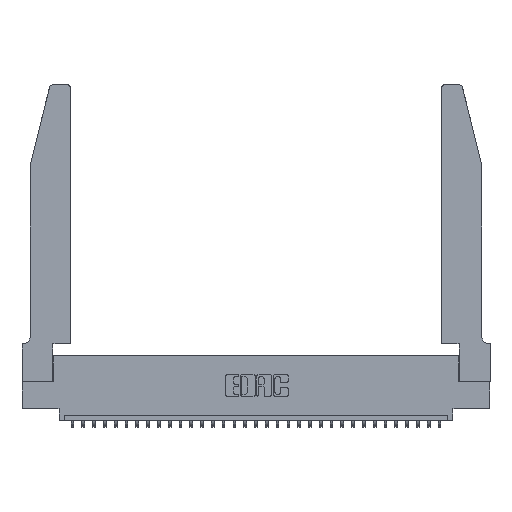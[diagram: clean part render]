
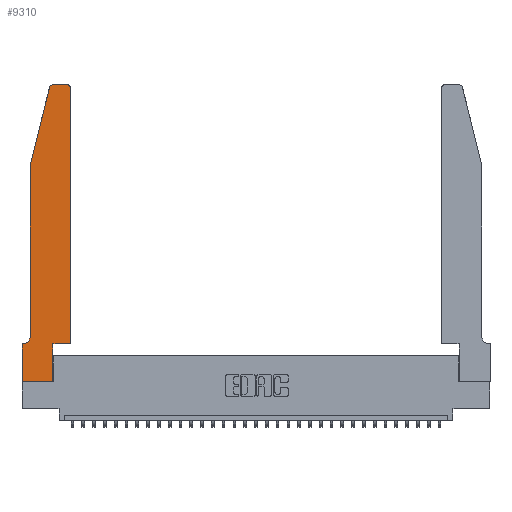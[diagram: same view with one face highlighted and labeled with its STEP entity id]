
A CAD part, top view. The second image highlights one B-rep face of the part: STEP entity #9310.
In plain terms, the highlighted planar face has unit normal (0, 0, 1).
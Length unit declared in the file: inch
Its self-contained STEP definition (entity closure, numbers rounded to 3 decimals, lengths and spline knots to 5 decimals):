
#14 = VECTOR ( 'NONE', #10910, 39.37008 ) ;
#64 = ORIENTED_EDGE ( 'NONE', *, *, #22052, .T. ) ;
#256 = VECTOR ( 'NONE', #29884, 39.37008 ) ;
#927 = DIRECTION ( 'NONE',  ( 0., 0., 1. ) ) ;
#1383 = CARTESIAN_POINT ( 'NONE',  ( 0.2865, 0.35, 0.37 ) ) ;
#1399 = VERTEX_POINT ( 'NONE', #5972 ) ;
#1616 = LINE ( 'NONE', #5135, #14 ) ;
#1634 = DIRECTION ( 'NONE',  ( -1., 0., 0. ) ) ;
#2352 = CARTESIAN_POINT ( 'NONE',  ( 0.4505, 0.35, 0.37 ) ) ;
#2363 = CIRCLE ( 'NONE', #27109, 0.03 ) ;
#3138 = CARTESIAN_POINT ( 'NONE',  ( 0.284, 2.72, 0.37 ) ) ;
#3613 = LINE ( 'NONE', #29501, #25014 ) ;
#3789 = EDGE_CURVE ( 'NONE', #22266, #21810, #1616, .T. ) ;
#3827 = DIRECTION ( 'NONE',  ( 1., 0., 0. ) ) ;
#4309 = DIRECTION ( 'NONE',  ( -0.239, -0.971, 0. ) ) ;
#4801 = EDGE_CURVE ( 'NONE', #29992, #10703, #20539, .T. ) ;
#4888 = ORIENTED_EDGE ( 'NONE', *, *, #19035, .T. ) ;
#5135 = CARTESIAN_POINT ( 'NONE',  ( 0., 0., 0.37 ) ) ;
#5917 = EDGE_CURVE ( 'NONE', #11358, #22266, #29902, .T. ) ;
#5972 = CARTESIAN_POINT ( 'NONE',  ( 0.4205, 2.75, 0.37 ) ) ;
#6533 = PLANE ( 'NONE',  #6714 ) ;
#6714 = AXIS2_PLACEMENT_3D ( 'NONE', #22581, #12165, #31314 ) ;
#6719 = DIRECTION ( 'NONE',  ( 0., 1., 0. ) ) ;
#6916 = LINE ( 'NONE', #19185, #27170 ) ;
#7336 = VECTOR ( 'NONE', #11769, 39.37008 ) ;
#7868 = CARTESIAN_POINT ( 'NONE',  ( 0., 0.35, 0.37 ) ) ;
#7906 = CARTESIAN_POINT ( 'NONE',  ( 0.4505, 2.72, 0.37 ) ) ;
#8883 = VECTOR ( 'NONE', #14076, 39.37008 ) ;
#8954 = DIRECTION ( 'NONE',  ( 0., -1., 0. ) ) ;
#9310 = ADVANCED_FACE ( 'NONE', ( #24325 ), #6533, .T. ) ;
#9419 = AXIS2_PLACEMENT_3D ( 'NONE', #23143, #927, #17660 ) ;
#9801 = EDGE_CURVE ( 'NONE', #23943, #29992, #13382, .T. ) ;
#10055 = EDGE_CURVE ( 'NONE', #10703, #16875, #3613, .T. ) ;
#10142 = VERTEX_POINT ( 'NONE', #15430 ) ;
#10177 = EDGE_CURVE ( 'NONE', #16875, #1399, #25815, .T. ) ;
#10609 = VERTEX_POINT ( 'NONE', #20280 ) ;
#10703 = VERTEX_POINT ( 'NONE', #27568 ) ;
#10845 = VERTEX_POINT ( 'NONE', #14107 ) ;
#10910 = DIRECTION ( 'NONE',  ( 0., -1., 0. ) ) ;
#11358 = VERTEX_POINT ( 'NONE', #20795 ) ;
#11662 = CARTESIAN_POINT ( 'NONE',  ( 0., 0., 0.37 ) ) ;
#11769 = DIRECTION ( 'NONE',  ( 1., 0., 0. ) ) ;
#12165 = DIRECTION ( 'NONE',  ( 0., 0., 1. ) ) ;
#13095 = EDGE_CURVE ( 'NONE', #10845, #20611, #27970, .T. ) ;
#13382 = LINE ( 'NONE', #1383, #29356 ) ;
#13859 = DIRECTION ( 'NONE',  ( 0., 0., -1. ) ) ;
#14076 = DIRECTION ( 'NONE',  ( 1., 0., 0. ) ) ;
#14107 = CARTESIAN_POINT ( 'NONE',  ( 0.0755, 2., 0.37 ) ) ;
#15074 = EDGE_CURVE ( 'NONE', #21810, #23943, #16726, .T. ) ;
#15115 = EDGE_CURVE ( 'NONE', #1399, #10142, #25945, .T. ) ;
#15430 = CARTESIAN_POINT ( 'NONE',  ( 0.284, 2.75, 0.37 ) ) ;
#16039 = ORIENTED_EDGE ( 'NONE', *, *, #4801, .T. ) ;
#16504 = ORIENTED_EDGE ( 'NONE', *, *, #9801, .T. ) ;
#16633 = CARTESIAN_POINT ( 'NONE',  ( 0.2605, 2.75, 0.37 ) ) ;
#16726 = LINE ( 'NONE', #11662, #8883 ) ;
#16875 = VERTEX_POINT ( 'NONE', #7906 ) ;
#17003 = CARTESIAN_POINT ( 'NONE',  ( 0.0755, 0.42, 0.37 ) ) ;
#17660 = DIRECTION ( 'NONE',  ( 1., 0., 0. ) ) ;
#18027 = EDGE_CURVE ( 'NONE', #20611, #11358, #19922, .T. ) ;
#18876 = ORIENTED_EDGE ( 'NONE', *, *, #15074, .T. ) ;
#19035 = EDGE_CURVE ( 'NONE', #10142, #10609, #2363, .T. ) ;
#19185 = CARTESIAN_POINT ( 'NONE',  ( 0.0755, 2., 0.37 ) ) ;
#19388 = ORIENTED_EDGE ( 'NONE', *, *, #13095, .T. ) ;
#19745 = DIRECTION ( 'NONE',  ( 0., 1., 0. ) ) ;
#19922 = CIRCLE ( 'NONE', #31297, 0.07 ) ;
#20088 = ORIENTED_EDGE ( 'NONE', *, *, #10177, .T. ) ;
#20280 = CARTESIAN_POINT ( 'NONE',  ( 0.25487, 2.72718, 0.37 ) ) ;
#20517 = CARTESIAN_POINT ( 'NONE',  ( 0.2865, 0.35, 0.37 ) ) ;
#20539 = LINE ( 'NONE', #2352, #7336 ) ;
#20601 = ORIENTED_EDGE ( 'NONE', *, *, #15115, .T. ) ;
#20611 = VERTEX_POINT ( 'NONE', #17003 ) ;
#20795 = CARTESIAN_POINT ( 'NONE',  ( 0.0055, 0.35, 0.37 ) ) ;
#21810 = VERTEX_POINT ( 'NONE', #31147 ) ;
#22002 = EDGE_LOOP ( 'NONE', ( #20601, #4888, #64, #19388, #27005, #27309, #24271, #18876, #16504, #16039, #24239, #20088 ) ) ;
#22052 = EDGE_CURVE ( 'NONE', #10609, #10845, #6916, .T. ) ;
#22266 = VERTEX_POINT ( 'NONE', #7868 ) ;
#22350 = CARTESIAN_POINT ( 'NONE',  ( 0.0755, 0.35, 0.37 ) ) ;
#22581 = CARTESIAN_POINT ( 'NONE',  ( 0., 0.35, 0.37 ) ) ;
#23073 = DIRECTION ( 'NONE',  ( 0., 0., 1. ) ) ;
#23143 = CARTESIAN_POINT ( 'NONE',  ( 0.4205, 2.72, 0.37 ) ) ;
#23943 = VERTEX_POINT ( 'NONE', #25048 ) ;
#24050 = DIRECTION ( 'NONE',  ( -1., 0., 0. ) ) ;
#24239 = ORIENTED_EDGE ( 'NONE', *, *, #10055, .T. ) ;
#24271 = ORIENTED_EDGE ( 'NONE', *, *, #3789, .T. ) ;
#24325 = FACE_OUTER_BOUND ( 'NONE', #22002, .T. ) ;
#25014 = VECTOR ( 'NONE', #19745, 39.37008 ) ;
#25048 = CARTESIAN_POINT ( 'NONE',  ( 0.2865, 0., 0.37 ) ) ;
#25571 = CARTESIAN_POINT ( 'NONE',  ( 0.0755, 2., 0.37 ) ) ;
#25815 = CIRCLE ( 'NONE', #9419, 0.03 ) ;
#25945 = LINE ( 'NONE', #16633, #29393 ) ;
#26418 = VECTOR ( 'NONE', #8954, 39.37008 ) ;
#27005 = ORIENTED_EDGE ( 'NONE', *, *, #18027, .T. ) ;
#27109 = AXIS2_PLACEMENT_3D ( 'NONE', #3138, #23073, #3827 ) ;
#27170 = VECTOR ( 'NONE', #4309, 39.37008 ) ;
#27309 = ORIENTED_EDGE ( 'NONE', *, *, #5917, .T. ) ;
#27568 = CARTESIAN_POINT ( 'NONE',  ( 0.4505, 0.35, 0.37 ) ) ;
#27970 = LINE ( 'NONE', #25571, #26418 ) ;
#28733 = CARTESIAN_POINT ( 'NONE',  ( 0.0055, 0.42, 0.37 ) ) ;
#29356 = VECTOR ( 'NONE', #6719, 39.37008 ) ;
#29393 = VECTOR ( 'NONE', #1634, 39.37008 ) ;
#29501 = CARTESIAN_POINT ( 'NONE',  ( 0.4505, 0.35, 0.37 ) ) ;
#29884 = DIRECTION ( 'NONE',  ( -1., 0., 0. ) ) ;
#29902 = LINE ( 'NONE', #22350, #256 ) ;
#29992 = VERTEX_POINT ( 'NONE', #20517 ) ;
#31147 = CARTESIAN_POINT ( 'NONE',  ( 0., 0., 0.37 ) ) ;
#31297 = AXIS2_PLACEMENT_3D ( 'NONE', #28733, #13859, #24050 ) ;
#31314 = DIRECTION ( 'NONE',  ( 1., 0., 0. ) ) ;
